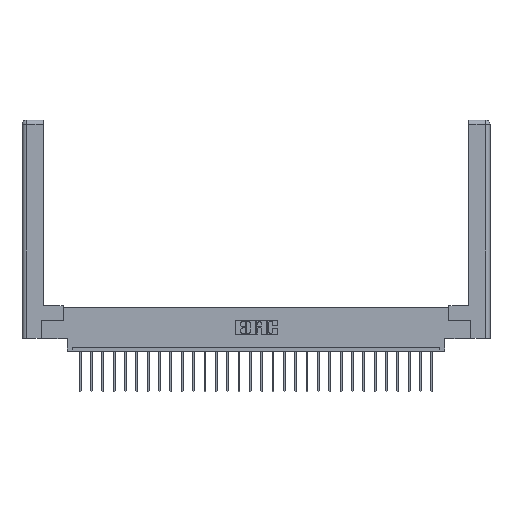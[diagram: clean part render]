
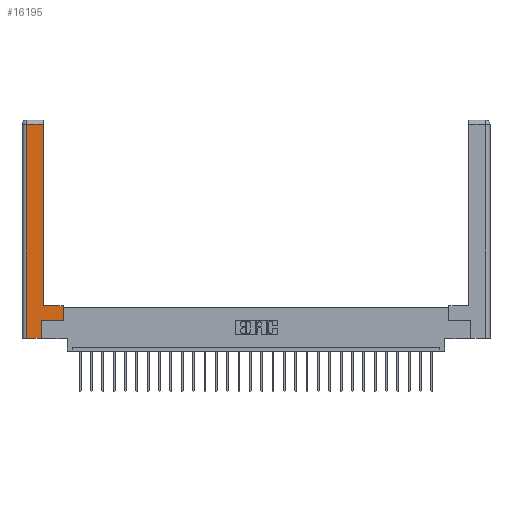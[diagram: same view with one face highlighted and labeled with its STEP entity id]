
A CAD part, top view. The second image highlights one B-rep face of the part: STEP entity #16195.
In plain terms, the highlighted planar face has unit normal (0, 0, 1).
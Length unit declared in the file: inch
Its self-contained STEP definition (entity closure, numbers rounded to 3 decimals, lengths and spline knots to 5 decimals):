
#454 = DIRECTION ( 'NONE',  ( 0., 1., 0. ) ) ;
#557 = VERTEX_POINT ( 'NONE', #24396 ) ;
#911 = VECTOR ( 'NONE', #6296, 39.37008 ) ;
#1044 = LINE ( 'NONE', #3675, #23231 ) ;
#1449 = VERTEX_POINT ( 'NONE', #16118 ) ;
#1498 = ORIENTED_EDGE ( 'NONE', *, *, #22892, .T. ) ;
#2722 = VECTOR ( 'NONE', #22989, 39.37008 ) ;
#3138 = LINE ( 'NONE', #20130, #11204 ) ;
#3675 = CARTESIAN_POINT ( 'NONE',  ( 0.295, 0.45, 0. ) ) ;
#4197 = EDGE_CURVE ( 'NONE', #10363, #6616, #6302, .T. ) ;
#4336 = LINE ( 'NONE', #9091, #15748 ) ;
#4729 = CARTESIAN_POINT ( 'NONE',  ( 0.0615, 2.94, 0. ) ) ;
#4838 = DIRECTION ( 'NONE',  ( -1., 0., 0. ) ) ;
#5195 = EDGE_CURVE ( 'NONE', #557, #1449, #4336, .T. ) ;
#6296 = DIRECTION ( 'NONE',  ( 1., 0., 0. ) ) ;
#6302 = LINE ( 'NONE', #25819, #911 ) ;
#6352 = LINE ( 'NONE', #17667, #15751 ) ;
#6616 = VERTEX_POINT ( 'NONE', #10346 ) ;
#7004 = CARTESIAN_POINT ( 'NONE',  ( 0.565, 0.45, 0. ) ) ;
#7585 = VERTEX_POINT ( 'NONE', #11691 ) ;
#7613 = CARTESIAN_POINT ( 'NONE',  ( 0.565, 0.245, 0. ) ) ;
#8625 = CARTESIAN_POINT ( 'NONE',  ( 0.0615, 0., 0. ) ) ;
#8641 = ORIENTED_EDGE ( 'NONE', *, *, #24355, .T. ) ;
#9091 = CARTESIAN_POINT ( 'NONE',  ( 0.295, 3., 0. ) ) ;
#9266 = EDGE_CURVE ( 'NONE', #7585, #27409, #23872, .T. ) ;
#9416 = ORIENTED_EDGE ( 'NONE', *, *, #5195, .T. ) ;
#10000 = ORIENTED_EDGE ( 'NONE', *, *, #26810, .T. ) ;
#10346 = CARTESIAN_POINT ( 'NONE',  ( 0.265, 0., 0. ) ) ;
#10363 = VERTEX_POINT ( 'NONE', #8625 ) ;
#11204 = VECTOR ( 'NONE', #11699, 39.37008 ) ;
#11344 = FACE_OUTER_BOUND ( 'NONE', #18640, .T. ) ;
#11597 = DIRECTION ( 'NONE',  ( 0., 0., -1. ) ) ;
#11691 = CARTESIAN_POINT ( 'NONE',  ( 0.265, 0.245, 0. ) ) ;
#11699 = DIRECTION ( 'NONE',  ( 0., 1., 0. ) ) ;
#11725 = CARTESIAN_POINT ( 'NONE',  ( 0.265, 0.245, 0. ) ) ;
#12084 = VECTOR ( 'NONE', #21321, 39.37008 ) ;
#13668 = DIRECTION ( 'NONE',  ( -1., 0., 0. ) ) ;
#14983 = CARTESIAN_POINT ( 'NONE',  ( 0.0615, 0., 0. ) ) ;
#15142 = ORIENTED_EDGE ( 'NONE', *, *, #4197, .T. ) ;
#15266 = EDGE_CURVE ( 'NONE', #1449, #27551, #6352, .T. ) ;
#15748 = VECTOR ( 'NONE', #454, 39.37008 ) ;
#15751 = VECTOR ( 'NONE', #4838, 39.37008 ) ;
#15960 = AXIS2_PLACEMENT_3D ( 'NONE', #24438, #11597, #13668 ) ;
#16118 = CARTESIAN_POINT ( 'NONE',  ( 0.295, 2.94, 0. ) ) ;
#16195 = ADVANCED_FACE ( 'NONE', ( #11344 ), #19664, .F. ) ;
#16793 = DIRECTION ( 'NONE',  ( -1., 0., 0. ) ) ;
#17211 = EDGE_CURVE ( 'NONE', #27409, #17685, #3138, .T. ) ;
#17667 = CARTESIAN_POINT ( 'NONE',  ( 0.0615, 2.94, 0. ) ) ;
#17685 = VERTEX_POINT ( 'NONE', #7004 ) ;
#18640 = EDGE_LOOP ( 'NONE', ( #9416, #26277, #8641, #15142, #10000, #22821, #23047, #1498 ) ) ;
#18666 = CARTESIAN_POINT ( 'NONE',  ( 0.565, 0.245, 0. ) ) ;
#19143 = LINE ( 'NONE', #14983, #12084 ) ;
#19664 = PLANE ( 'NONE',  #15960 ) ;
#20130 = CARTESIAN_POINT ( 'NONE',  ( 0.565, 0.45, 0. ) ) ;
#21321 = DIRECTION ( 'NONE',  ( 0., -1., 0. ) ) ;
#22584 = DIRECTION ( 'NONE',  ( 0., 1., 0. ) ) ;
#22821 = ORIENTED_EDGE ( 'NONE', *, *, #9266, .T. ) ;
#22892 = EDGE_CURVE ( 'NONE', #17685, #557, #1044, .T. ) ;
#22989 = DIRECTION ( 'NONE',  ( 1., 0., 0. ) ) ;
#23047 = ORIENTED_EDGE ( 'NONE', *, *, #17211, .T. ) ;
#23231 = VECTOR ( 'NONE', #16793, 39.37008 ) ;
#23872 = LINE ( 'NONE', #18666, #2722 ) ;
#24001 = LINE ( 'NONE', #11725, #25380 ) ;
#24355 = EDGE_CURVE ( 'NONE', #27551, #10363, #19143, .T. ) ;
#24396 = CARTESIAN_POINT ( 'NONE',  ( 0.295, 0.45, 0. ) ) ;
#24438 = CARTESIAN_POINT ( 'NONE',  ( 0., 0., 0. ) ) ;
#25380 = VECTOR ( 'NONE', #22584, 39.37008 ) ;
#25819 = CARTESIAN_POINT ( 'NONE',  ( 0.265, 0., 0. ) ) ;
#26277 = ORIENTED_EDGE ( 'NONE', *, *, #15266, .T. ) ;
#26810 = EDGE_CURVE ( 'NONE', #6616, #7585, #24001, .T. ) ;
#27409 = VERTEX_POINT ( 'NONE', #7613 ) ;
#27551 = VERTEX_POINT ( 'NONE', #4729 ) ;
